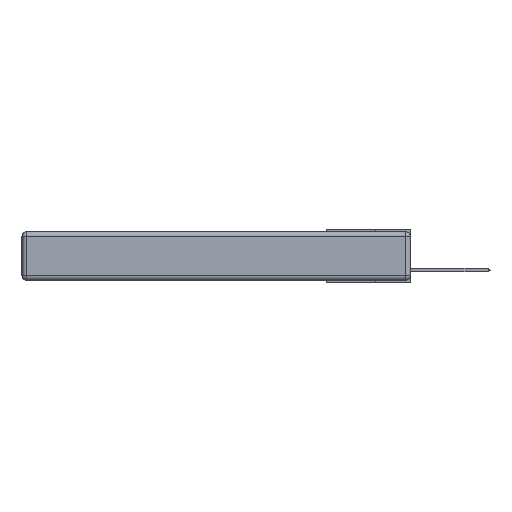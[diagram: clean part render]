
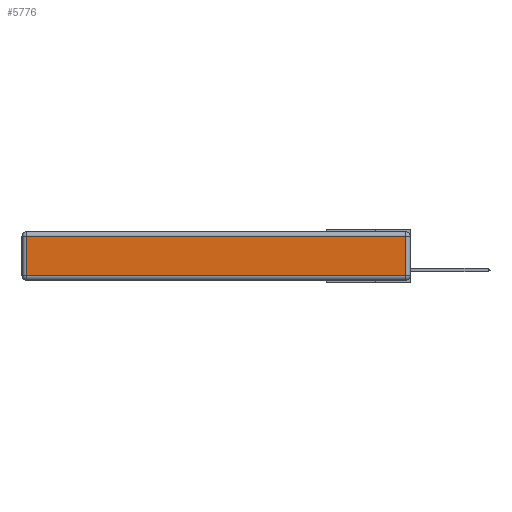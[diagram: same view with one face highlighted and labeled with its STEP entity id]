
A CAD part, left-side view. The second image highlights one B-rep face of the part: STEP entity #5776.
In plain terms, the highlighted planar face has unit normal (-1, 0, 0).
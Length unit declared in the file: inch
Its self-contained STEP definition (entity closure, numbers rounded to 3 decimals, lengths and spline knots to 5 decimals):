
#183 = DIRECTION ( 'NONE',  ( 0., 0., 1. ) ) ;
#1418 = CARTESIAN_POINT ( 'NONE',  ( 0., 2.72, -0.313 ) ) ;
#1524 = CARTESIAN_POINT ( 'NONE',  ( 0., 2.72, -0.343 ) ) ;
#1957 = DIRECTION ( 'NONE',  ( 0., -1., 0. ) ) ;
#2439 = LINE ( 'NONE', #16980, #15530 ) ;
#3213 = VERTEX_POINT ( 'NONE', #3323 ) ;
#3323 = CARTESIAN_POINT ( 'NONE',  ( 0., 2.72, -0.03 ) ) ;
#3882 = CARTESIAN_POINT ( 'NONE',  ( 0., 0., -0.313 ) ) ;
#3923 = AXIS2_PLACEMENT_3D ( 'NONE', #20475, #5303, #183 ) ;
#5303 = DIRECTION ( 'NONE',  ( -1., 0., 0. ) ) ;
#5480 = VECTOR ( 'NONE', #13122, 39.37008 ) ;
#5776 = ADVANCED_FACE ( 'NONE', ( #13738 ), #6942, .T. ) ;
#6942 = PLANE ( 'NONE',  #3923 ) ;
#7861 = ORIENTED_EDGE ( 'NONE', *, *, #10829, .T. ) ;
#9400 = VERTEX_POINT ( 'NONE', #15113 ) ;
#9836 = CARTESIAN_POINT ( 'NONE',  ( 0., 0.03, -0.03 ) ) ;
#10608 = VECTOR ( 'NONE', #18252, 39.37008 ) ;
#10829 = EDGE_CURVE ( 'NONE', #11563, #9400, #12698, .T. ) ;
#11563 = VERTEX_POINT ( 'NONE', #1418 ) ;
#12698 = LINE ( 'NONE', #3882, #20842 ) ;
#13122 = DIRECTION ( 'NONE',  ( 0., 1., 0. ) ) ;
#13615 = DIRECTION ( 'NONE',  ( 0., 0., 1. ) ) ;
#13738 = FACE_OUTER_BOUND ( 'NONE', #16263, .T. ) ;
#14586 = VERTEX_POINT ( 'NONE', #9836 ) ;
#14872 = ORIENTED_EDGE ( 'NONE', *, *, #21744, .T. ) ;
#15029 = LINE ( 'NONE', #1524, #10608 ) ;
#15113 = CARTESIAN_POINT ( 'NONE',  ( 0., 0.03, -0.313 ) ) ;
#15530 = VECTOR ( 'NONE', #13615, 39.37008 ) ;
#16263 = EDGE_LOOP ( 'NONE', ( #7861, #14872, #21146, #21592 ) ) ;
#16477 = LINE ( 'NONE', #19811, #5480 ) ;
#16980 = CARTESIAN_POINT ( 'NONE',  ( 0., 0.03, -0.343 ) ) ;
#18252 = DIRECTION ( 'NONE',  ( 0., 0., -1. ) ) ;
#19424 = EDGE_CURVE ( 'NONE', #14586, #3213, #16477, .T. ) ;
#19811 = CARTESIAN_POINT ( 'NONE',  ( 0., 2.75, -0.03 ) ) ;
#20475 = CARTESIAN_POINT ( 'NONE',  ( 0., 0., -0.343 ) ) ;
#20842 = VECTOR ( 'NONE', #1957, 39.37008 ) ;
#21146 = ORIENTED_EDGE ( 'NONE', *, *, #19424, .T. ) ;
#21592 = ORIENTED_EDGE ( 'NONE', *, *, #21614, .T. ) ;
#21614 = EDGE_CURVE ( 'NONE', #3213, #11563, #15029, .T. ) ;
#21744 = EDGE_CURVE ( 'NONE', #9400, #14586, #2439, .T. ) ;
